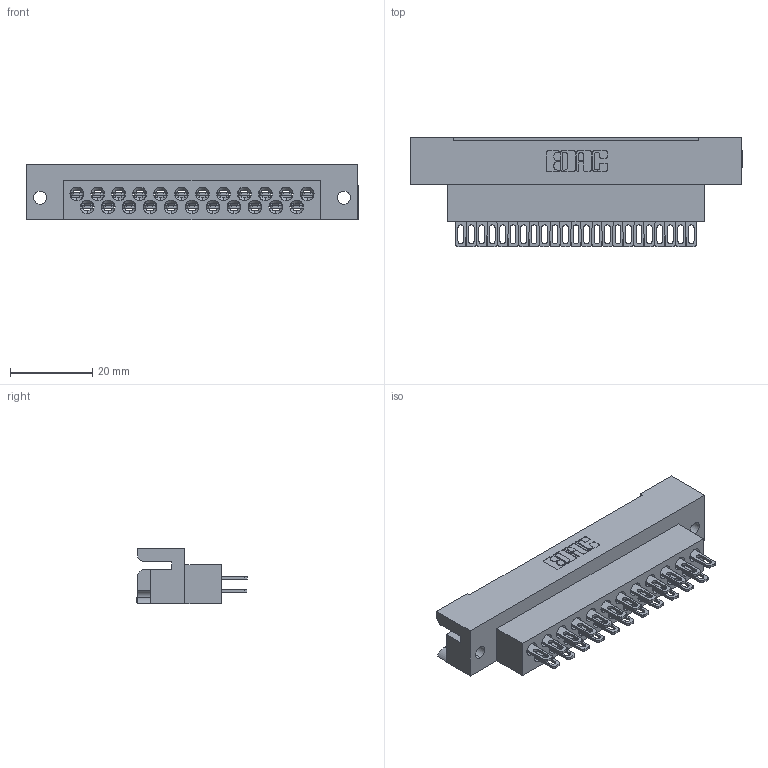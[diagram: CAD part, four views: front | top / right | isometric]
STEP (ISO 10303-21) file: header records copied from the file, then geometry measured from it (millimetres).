
FILE_DESCRIPTION (( 'STEP AP203' ), '1' );
FILE_NAME ('438-023-500-122.STEP', '2020-03-12T20:30:49', ( '' ), ( '' ), 'SwSTEP 2.0', 'SolidWorks 2016', '' );
FILE_SCHEMA (( 'CONFIG_CONTROL_DESIGN' ));
Length unit declared in the file: millimetre
Products named in the file (3): 516-290-001_500; 438-210-001_438-210-023-112; 438-023-500-122
Assembly tree (24 placements, depth 2):
  438-023-500-122
    438-210-001_438-210-023-112
    516-290-001_500  x23
Bounding box: 80.52 x 26.68 x 13.49 mm (x, y, z)
Volume: 12964.6 mm3; surface area: 15917.4 mm2
Topology: 24 solids, 24 shells, 2502 faces, 7290 edges, 4821 vertices
Faces by surface type: plane 1556, cylinder 717, bspline 160, cone 69
Entity records: 29907 total; most frequent: CARTESIAN_POINT 7115, ORIENTED_EDGE 4900, DIRECTION 4155, EDGE_CURVE 2450, LINE 1695, VECTOR 1695, VERTEX_POINT 1609, AXIS2_PLACEMENT_3D 1230
